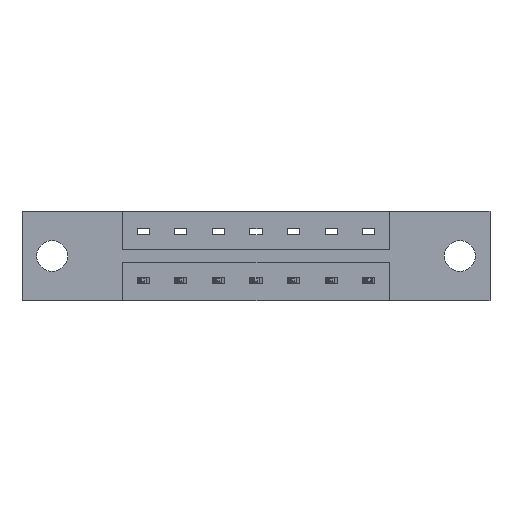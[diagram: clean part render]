
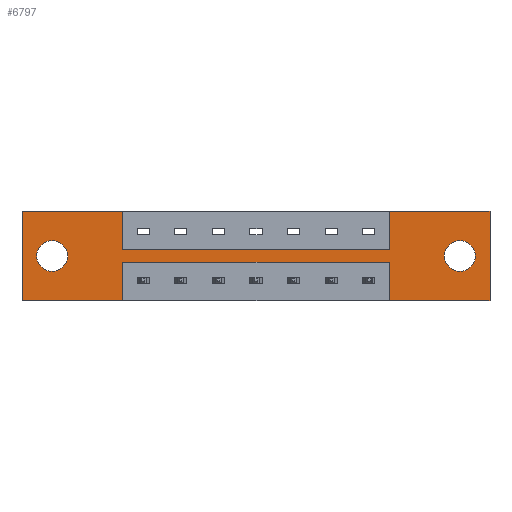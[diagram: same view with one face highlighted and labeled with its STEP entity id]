
A CAD part, front view. The second image highlights one B-rep face of the part: STEP entity #6797.
In plain terms, the highlighted planar face has unit normal (0, -1, 0).
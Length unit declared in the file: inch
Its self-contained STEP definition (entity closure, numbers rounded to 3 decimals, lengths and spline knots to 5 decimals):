
#106 = LINE ( 'NONE', #4793, #1575 ) ;
#151 = EDGE_LOOP ( 'NONE', ( #788, #2447 ) ) ;
#425 = VERTEX_POINT ( 'NONE', #6782 ) ;
#428 = CARTESIAN_POINT ( 'NONE',  ( 0.125, 0., -0.249 ) ) ;
#440 = LINE ( 'NONE', #3146, #6555 ) ;
#616 = LINE ( 'NONE', #5961, #4114 ) ;
#656 = VERTEX_POINT ( 'NONE', #7811 ) ;
#665 = DIRECTION ( 'NONE',  ( 0., 0., -1. ) ) ;
#788 = ORIENTED_EDGE ( 'NONE', *, *, #5102, .T. ) ;
#823 = DIRECTION ( 'NONE',  ( 0., 0., -1. ) ) ;
#963 = VERTEX_POINT ( 'NONE', #2749 ) ;
#989 = VECTOR ( 'NONE', #8189, 39.37008 ) ;
#1017 = EDGE_CURVE ( 'NONE', #4934, #5886, #2873, .T. ) ;
#1038 = AXIS2_PLACEMENT_3D ( 'NONE', #8245, #8168, #823 ) ;
#1132 = VERTEX_POINT ( 'NONE', #6794 ) ;
#1146 = VECTOR ( 'NONE', #6896, 39.37008 ) ;
#1378 = ORIENTED_EDGE ( 'NONE', *, *, #6891, .F. ) ;
#1408 = VERTEX_POINT ( 'NONE', #2335 ) ;
#1459 = DIRECTION ( 'NONE',  ( 0., 0., -1. ) ) ;
#1575 = VECTOR ( 'NONE', #1459, 39.37008 ) ;
#1627 = VERTEX_POINT ( 'NONE', #8300 ) ;
#1638 = VERTEX_POINT ( 'NONE', #2651 ) ;
#1657 = EDGE_CURVE ( 'NONE', #1638, #1408, #6934, .T. ) ;
#1660 = EDGE_CURVE ( 'NONE', #3178, #8734, #2877, .T. ) ;
#1664 = EDGE_CURVE ( 'NONE', #1627, #2263, #7607, .T. ) ;
#1745 = CIRCLE ( 'NONE', #8183, 0.064 ) ;
#1748 = EDGE_CURVE ( 'NONE', #425, #3025, #3412, .T. ) ;
#1796 = DIRECTION ( 'NONE',  ( 0., 0., 1. ) ) ;
#1998 = CARTESIAN_POINT ( 'NONE',  ( 0.125, 0., -0.121 ) ) ;
#2099 = CARTESIAN_POINT ( 'NONE',  ( 0.4175, 0., -0.1585 ) ) ;
#2105 = CARTESIAN_POINT ( 'NONE',  ( 1.5225, 0., -0.1585 ) ) ;
#2108 = CIRCLE ( 'NONE', #4694, 0.064 ) ;
#2127 = LINE ( 'NONE', #4867, #989 ) ;
#2228 = ORIENTED_EDGE ( 'NONE', *, *, #3608, .F. ) ;
#2251 = ORIENTED_EDGE ( 'NONE', *, *, #7458, .F. ) ;
#2263 = VERTEX_POINT ( 'NONE', #6382 ) ;
#2288 = CARTESIAN_POINT ( 'NONE',  ( 0., 0., -0.37 ) ) ;
#2320 = ORIENTED_EDGE ( 'NONE', *, *, #6950, .F. ) ;
#2335 = CARTESIAN_POINT ( 'NONE',  ( 1.5225, 0., 0. ) ) ;
#2447 = ORIENTED_EDGE ( 'NONE', *, *, #1660, .T. ) ;
#2462 = DIRECTION ( 'NONE',  ( 0., 0., -1. ) ) ;
#2651 = CARTESIAN_POINT ( 'NONE',  ( 1.5225, 0., -0.1585 ) ) ;
#2749 = CARTESIAN_POINT ( 'NONE',  ( 1.94, 0., 0. ) ) ;
#2777 = DIRECTION ( 'NONE',  ( 0., 1., 0. ) ) ;
#2873 = LINE ( 'NONE', #8503, #6877 ) ;
#2877 = CIRCLE ( 'NONE', #7172, 0.064 ) ;
#2911 = EDGE_CURVE ( 'NONE', #2263, #1627, #2108, .T. ) ;
#2955 = FACE_BOUND ( 'NONE', #3643, .T. ) ;
#3025 = VERTEX_POINT ( 'NONE', #8418 ) ;
#3048 = DIRECTION ( 'NONE',  ( 0., -1., 0. ) ) ;
#3146 = CARTESIAN_POINT ( 'NONE',  ( 0., 0., 0. ) ) ;
#3178 = VERTEX_POINT ( 'NONE', #428 ) ;
#3180 = CARTESIAN_POINT ( 'NONE',  ( 0.125, 0., -0.185 ) ) ;
#3181 = DIRECTION ( 'NONE',  ( -1., 0., 0. ) ) ;
#3268 = DIRECTION ( 'NONE',  ( 0., 1., 0. ) ) ;
#3367 = CARTESIAN_POINT ( 'NONE',  ( 0., 0., 0. ) ) ;
#3412 = LINE ( 'NONE', #6768, #6601 ) ;
#3535 = LINE ( 'NONE', #4175, #6702 ) ;
#3551 = VERTEX_POINT ( 'NONE', #6680 ) ;
#3608 = EDGE_CURVE ( 'NONE', #1132, #5986, #440, .T. ) ;
#3643 = EDGE_LOOP ( 'NONE', ( #8177, #7980 ) ) ;
#3713 = EDGE_CURVE ( 'NONE', #3025, #4070, #3535, .T. ) ;
#3859 = CARTESIAN_POINT ( 'NONE',  ( 1.94, 0., 0. ) ) ;
#4070 = VERTEX_POINT ( 'NONE', #4194 ) ;
#4114 = VECTOR ( 'NONE', #3181, 39.37008 ) ;
#4172 = CARTESIAN_POINT ( 'NONE',  ( 0.125, 0., -0.185 ) ) ;
#4174 = CARTESIAN_POINT ( 'NONE',  ( 1.815, 0., -0.185 ) ) ;
#4175 = CARTESIAN_POINT ( 'NONE',  ( 0., 0., -0.37 ) ) ;
#4194 = CARTESIAN_POINT ( 'NONE',  ( 0., 0., -0.37 ) ) ;
#4255 = DIRECTION ( 'NONE',  ( 1., 0., 0. ) ) ;
#4346 = LINE ( 'NONE', #8513, #6969 ) ;
#4404 = VECTOR ( 'NONE', #2462, 39.37008 ) ;
#4647 = CARTESIAN_POINT ( 'NONE',  ( 0.4175, 0., 0. ) ) ;
#4694 = AXIS2_PLACEMENT_3D ( 'NONE', #4174, #2777, #8211 ) ;
#4793 = CARTESIAN_POINT ( 'NONE',  ( 0.4175, 0., -0.1585 ) ) ;
#4864 = ORIENTED_EDGE ( 'NONE', *, *, #1748, .F. ) ;
#4867 = CARTESIAN_POINT ( 'NONE',  ( 0., 0., 0. ) ) ;
#4934 = VERTEX_POINT ( 'NONE', #8306 ) ;
#5070 = FACE_OUTER_BOUND ( 'NONE', #7428, .T. ) ;
#5102 = EDGE_CURVE ( 'NONE', #8734, #3178, #1745, .T. ) ;
#5301 = ORIENTED_EDGE ( 'NONE', *, *, #1017, .F. ) ;
#5311 = EDGE_CURVE ( 'NONE', #1408, #963, #6938, .T. ) ;
#5510 = DIRECTION ( 'NONE',  ( 0., 1., 0. ) ) ;
#5574 = ORIENTED_EDGE ( 'NONE', *, *, #3713, .F. ) ;
#5695 = DIRECTION ( 'NONE',  ( -1., 0., 0. ) ) ;
#5886 = VERTEX_POINT ( 'NONE', #7653 ) ;
#5891 = VECTOR ( 'NONE', #7623, 39.37008 ) ;
#5961 = CARTESIAN_POINT ( 'NONE',  ( 0.4175, 0., -0.2115 ) ) ;
#5986 = VERTEX_POINT ( 'NONE', #4647 ) ;
#6290 = ORIENTED_EDGE ( 'NONE', *, *, #7776, .F. ) ;
#6359 = ORIENTED_EDGE ( 'NONE', *, *, #6824, .F. ) ;
#6382 = CARTESIAN_POINT ( 'NONE',  ( 1.815, 0., -0.121 ) ) ;
#6528 = DIRECTION ( 'NONE',  ( 0., 0., 1. ) ) ;
#6531 = ORIENTED_EDGE ( 'NONE', *, *, #7845, .F. ) ;
#6555 = VECTOR ( 'NONE', #6597, 39.37008 ) ;
#6597 = DIRECTION ( 'NONE',  ( 1., 0., 0. ) ) ;
#6601 = VECTOR ( 'NONE', #665, 39.37008 ) ;
#6680 = CARTESIAN_POINT ( 'NONE',  ( 1.94, 0., -0.37 ) ) ;
#6702 = VECTOR ( 'NONE', #6860, 39.37008 ) ;
#6768 = CARTESIAN_POINT ( 'NONE',  ( 0.4175, 0., -0.2115 ) ) ;
#6782 = CARTESIAN_POINT ( 'NONE',  ( 0.4175, 0., -0.2115 ) ) ;
#6794 = CARTESIAN_POINT ( 'NONE',  ( 0., 0., 0. ) ) ;
#6797 = ADVANCED_FACE ( 'NONE', ( #2955, #8471, #5070 ), #7217, .T. ) ;
#6824 = EDGE_CURVE ( 'NONE', #3551, #4934, #4346, .T. ) ;
#6860 = DIRECTION ( 'NONE',  ( -1., 0., 0. ) ) ;
#6877 = VECTOR ( 'NONE', #6528, 39.37008 ) ;
#6891 = EDGE_CURVE ( 'NONE', #5886, #425, #616, .T. ) ;
#6896 = DIRECTION ( 'NONE',  ( 1., 0., 0. ) ) ;
#6934 = LINE ( 'NONE', #2105, #5891 ) ;
#6938 = LINE ( 'NONE', #3367, #8460 ) ;
#6950 = EDGE_CURVE ( 'NONE', #963, #3551, #8752, .T. ) ;
#6969 = VECTOR ( 'NONE', #5695, 39.37008 ) ;
#7172 = AXIS2_PLACEMENT_3D ( 'NONE', #4172, #5510, #7452 ) ;
#7217 = PLANE ( 'NONE',  #7550 ) ;
#7313 = ORIENTED_EDGE ( 'NONE', *, *, #5311, .F. ) ;
#7428 = EDGE_LOOP ( 'NONE', ( #5301, #6359, #2320, #7313, #7880, #6531, #6290, #2228, #2251, #5574, #4864, #1378 ) ) ;
#7452 = DIRECTION ( 'NONE',  ( 0., 0., 1. ) ) ;
#7458 = EDGE_CURVE ( 'NONE', #4070, #1132, #2127, .T. ) ;
#7550 = AXIS2_PLACEMENT_3D ( 'NONE', #2288, #3048, #7765 ) ;
#7607 = CIRCLE ( 'NONE', #1038, 0.064 ) ;
#7623 = DIRECTION ( 'NONE',  ( 0., 0., 1. ) ) ;
#7653 = CARTESIAN_POINT ( 'NONE',  ( 1.5225, 0., -0.2115 ) ) ;
#7765 = DIRECTION ( 'NONE',  ( 0., 0., -1. ) ) ;
#7776 = EDGE_CURVE ( 'NONE', #5986, #656, #106, .T. ) ;
#7811 = CARTESIAN_POINT ( 'NONE',  ( 0.4175, 0., -0.1585 ) ) ;
#7845 = EDGE_CURVE ( 'NONE', #656, #1638, #8242, .T. ) ;
#7880 = ORIENTED_EDGE ( 'NONE', *, *, #1657, .F. ) ;
#7980 = ORIENTED_EDGE ( 'NONE', *, *, #1664, .T. ) ;
#8168 = DIRECTION ( 'NONE',  ( 0., 1., 0. ) ) ;
#8177 = ORIENTED_EDGE ( 'NONE', *, *, #2911, .T. ) ;
#8183 = AXIS2_PLACEMENT_3D ( 'NONE', #3180, #3268, #1796 ) ;
#8189 = DIRECTION ( 'NONE',  ( 0., 0., 1. ) ) ;
#8211 = DIRECTION ( 'NONE',  ( 0., 0., -1. ) ) ;
#8242 = LINE ( 'NONE', #2099, #1146 ) ;
#8245 = CARTESIAN_POINT ( 'NONE',  ( 1.815, 0., -0.185 ) ) ;
#8300 = CARTESIAN_POINT ( 'NONE',  ( 1.815, 0., -0.249 ) ) ;
#8306 = CARTESIAN_POINT ( 'NONE',  ( 1.5225, 0., -0.37 ) ) ;
#8418 = CARTESIAN_POINT ( 'NONE',  ( 0.4175, 0., -0.37 ) ) ;
#8460 = VECTOR ( 'NONE', #4255, 39.37008 ) ;
#8471 = FACE_BOUND ( 'NONE', #151, .T. ) ;
#8503 = CARTESIAN_POINT ( 'NONE',  ( 1.5225, 0., -0.2115 ) ) ;
#8513 = CARTESIAN_POINT ( 'NONE',  ( 0., 0., -0.37 ) ) ;
#8734 = VERTEX_POINT ( 'NONE', #1998 ) ;
#8752 = LINE ( 'NONE', #3859, #4404 ) ;
